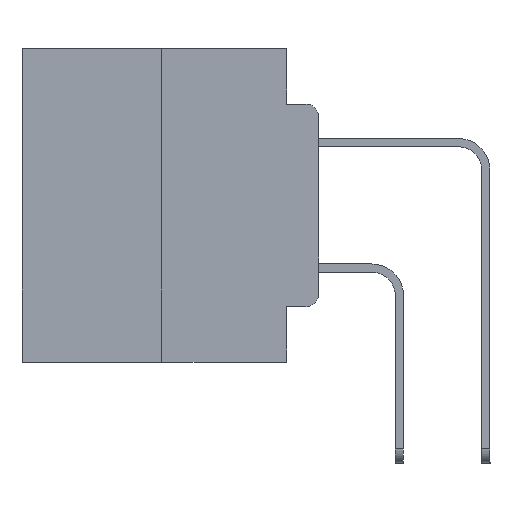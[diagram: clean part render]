
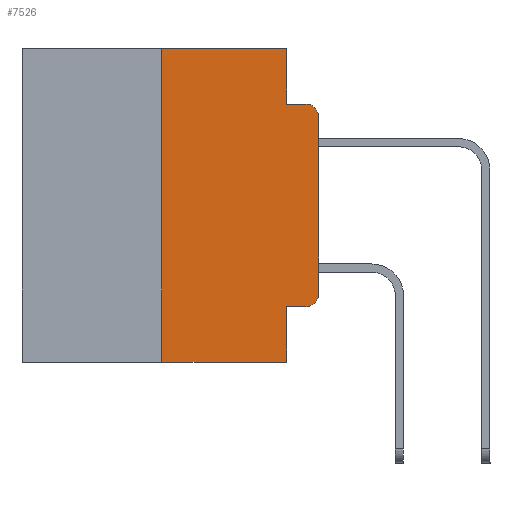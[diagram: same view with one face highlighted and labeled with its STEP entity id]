
A CAD part, left-side view. The second image highlights one B-rep face of the part: STEP entity #7526.
In plain terms, the highlighted planar face has unit normal (-1, 0, 0).
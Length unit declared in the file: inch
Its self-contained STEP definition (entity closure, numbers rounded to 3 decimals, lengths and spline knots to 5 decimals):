
#521 = LINE ( 'NONE', #25987, #11988 ) ;
#642 = DIRECTION ( 'NONE',  ( 0., -1., 0. ) ) ;
#853 = VECTOR ( 'NONE', #24153, 39.37008 ) ;
#867 = ORIENTED_EDGE ( 'NONE', *, *, #5692, .T. ) ;
#997 = ORIENTED_EDGE ( 'NONE', *, *, #10166, .F. ) ;
#1089 = ORIENTED_EDGE ( 'NONE', *, *, #15028, .T. ) ;
#1192 = DIRECTION ( 'NONE',  ( 0., 0., -1. ) ) ;
#1322 = ORIENTED_EDGE ( 'NONE', *, *, #11628, .F. ) ;
#1392 = ORIENTED_EDGE ( 'NONE', *, *, #2798, .F. ) ;
#1606 = ORIENTED_EDGE ( 'NONE', *, *, #13150, .F. ) ;
#1665 = ORIENTED_EDGE ( 'NONE', *, *, #16077, .F. ) ;
#2149 = ORIENTED_EDGE ( 'NONE', *, *, #17499, .T. ) ;
#2210 = ORIENTED_EDGE ( 'NONE', *, *, #18893, .T. ) ;
#2421 = LINE ( 'NONE', #17740, #853 ) ;
#2798 = EDGE_CURVE ( 'NONE', #20908, #28083, #6882, .T. ) ;
#2975 = CARTESIAN_POINT ( 'NONE',  ( 0., 0.25, -0.5 ) ) ;
#3703 = VERTEX_POINT ( 'NONE', #20755 ) ;
#3788 = DIRECTION ( 'NONE',  ( 0., 0., -1. ) ) ;
#4156 = EDGE_CURVE ( 'NONE', #19095, #19832, #26447, .T. ) ;
#4952 = CARTESIAN_POINT ( 'NONE',  ( 0., 0.25, 0. ) ) ;
#5104 = CARTESIAN_POINT ( 'NONE',  ( 0., 0.25, 0. ) ) ;
#5175 = CARTESIAN_POINT ( 'NONE',  ( 0., 0.051, -0.5 ) ) ;
#5692 = EDGE_CURVE ( 'NONE', #3703, #19095, #2421, .T. ) ;
#6221 = DIRECTION ( 'NONE',  ( 0., 0., -1. ) ) ;
#6882 = LINE ( 'NONE', #9634, #17849 ) ;
#6973 = LINE ( 'NONE', #5104, #23583 ) ;
#7294 = AXIS2_PLACEMENT_3D ( 'NONE', #21085, #14799, #1192 ) ;
#7345 = VERTEX_POINT ( 'NONE', #5175 ) ;
#7526 = ADVANCED_FACE ( 'NONE', ( #25612 ), #23240, .F. ) ;
#7757 = VECTOR ( 'NONE', #23321, 39.37008 ) ;
#7940 = LINE ( 'NONE', #10584, #24484 ) ;
#9067 = CARTESIAN_POINT ( 'NONE',  ( 0., 0.02, -0.4115 ) ) ;
#9257 = DIRECTION ( 'NONE',  ( 0., -1., 0. ) ) ;
#9520 = EDGE_LOOP ( 'NONE', ( #2210, #2149, #1665, #1606, #1392, #1322, #1089, #997, #867, #11699 ) ) ;
#9634 = CARTESIAN_POINT ( 'NONE',  ( 0., 0.473, 0. ) ) ;
#10166 = EDGE_CURVE ( 'NONE', #3703, #7345, #26325, .T. ) ;
#10584 = CARTESIAN_POINT ( 'NONE',  ( 0., 0.051, 0. ) ) ;
#11426 = CARTESIAN_POINT ( 'NONE',  ( 0., 0.02, -0.0885 ) ) ;
#11628 = EDGE_CURVE ( 'NONE', #24644, #20908, #6973, .T. ) ;
#11699 = ORIENTED_EDGE ( 'NONE', *, *, #4156, .T. ) ;
#11988 = VECTOR ( 'NONE', #28091, 39.37008 ) ;
#12143 = CARTESIAN_POINT ( 'NONE',  ( 0., 0.051, -0.0885 ) ) ;
#12305 = CARTESIAN_POINT ( 'NONE',  ( 0., 0.02, -0.1085 ) ) ;
#13150 = EDGE_CURVE ( 'NONE', #28083, #22104, #7940, .T. ) ;
#13630 = LINE ( 'NONE', #25551, #7757 ) ;
#14578 = DIRECTION ( 'NONE',  ( 0., 0., -1. ) ) ;
#14799 = DIRECTION ( 'NONE',  ( 1., 0., 0. ) ) ;
#14879 = VERTEX_POINT ( 'NONE', #14960 ) ;
#14960 = CARTESIAN_POINT ( 'NONE',  ( 0., 0., -0.1085 ) ) ;
#15028 = EDGE_CURVE ( 'NONE', #24644, #7345, #521, .T. ) ;
#15054 = VECTOR ( 'NONE', #3788, 39.37008 ) ;
#15449 = AXIS2_PLACEMENT_3D ( 'NONE', #12305, #27260, #14578 ) ;
#16077 = EDGE_CURVE ( 'NONE', #22104, #17880, #26162, .T. ) ;
#17079 = CARTESIAN_POINT ( 'NONE',  ( 0., 0.051, 0. ) ) ;
#17499 = EDGE_CURVE ( 'NONE', #14879, #17880, #21425, .T. ) ;
#17740 = CARTESIAN_POINT ( 'NONE',  ( 0., 0.051, -0.4115 ) ) ;
#17849 = VECTOR ( 'NONE', #9257, 39.37008 ) ;
#17880 = VERTEX_POINT ( 'NONE', #11426 ) ;
#18893 = EDGE_CURVE ( 'NONE', #19832, #14879, #13630, .T. ) ;
#19095 = VERTEX_POINT ( 'NONE', #9067 ) ;
#19832 = VERTEX_POINT ( 'NONE', #26607 ) ;
#20447 = CARTESIAN_POINT ( 'NONE',  ( 0., 0.051, 0. ) ) ;
#20755 = CARTESIAN_POINT ( 'NONE',  ( 0., 0.051, -0.4115 ) ) ;
#20908 = VERTEX_POINT ( 'NONE', #4952 ) ;
#21066 = AXIS2_PLACEMENT_3D ( 'NONE', #21264, #23576, #23221 ) ;
#21085 = CARTESIAN_POINT ( 'NONE',  ( 0., 0.473, 0. ) ) ;
#21264 = CARTESIAN_POINT ( 'NONE',  ( 0., 0.02, -0.3915 ) ) ;
#21425 = CIRCLE ( 'NONE', #15449, 0.02 ) ;
#22104 = VERTEX_POINT ( 'NONE', #28252 ) ;
#23221 = DIRECTION ( 'NONE',  ( 0., 0., -1. ) ) ;
#23240 = PLANE ( 'NONE',  #7294 ) ;
#23321 = DIRECTION ( 'NONE',  ( 0., 0., 1. ) ) ;
#23576 = DIRECTION ( 'NONE',  ( -1., 0., 0. ) ) ;
#23583 = VECTOR ( 'NONE', #24647, 39.37008 ) ;
#24153 = DIRECTION ( 'NONE',  ( 0., -1., 0. ) ) ;
#24484 = VECTOR ( 'NONE', #6221, 39.37008 ) ;
#24644 = VERTEX_POINT ( 'NONE', #2975 ) ;
#24647 = DIRECTION ( 'NONE',  ( 0., 0., 1. ) ) ;
#25494 = VECTOR ( 'NONE', #642, 39.37008 ) ;
#25551 = CARTESIAN_POINT ( 'NONE',  ( 0., 0., 0. ) ) ;
#25612 = FACE_OUTER_BOUND ( 'NONE', #9520, .T. ) ;
#25987 = CARTESIAN_POINT ( 'NONE',  ( 0., 0.473, -0.5 ) ) ;
#26162 = LINE ( 'NONE', #12143, #25494 ) ;
#26325 = LINE ( 'NONE', #17079, #15054 ) ;
#26447 = CIRCLE ( 'NONE', #21066, 0.02 ) ;
#26607 = CARTESIAN_POINT ( 'NONE',  ( 0., 0., -0.3915 ) ) ;
#27260 = DIRECTION ( 'NONE',  ( -1., 0., 0. ) ) ;
#28083 = VERTEX_POINT ( 'NONE', #20447 ) ;
#28091 = DIRECTION ( 'NONE',  ( 0., -1., 0. ) ) ;
#28252 = CARTESIAN_POINT ( 'NONE',  ( 0., 0.051, -0.0885 ) ) ;
